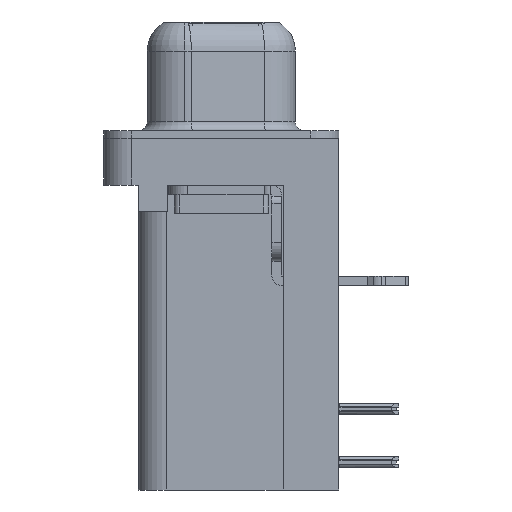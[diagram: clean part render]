
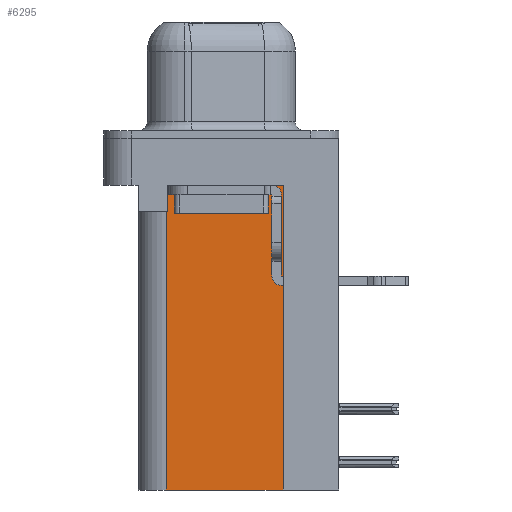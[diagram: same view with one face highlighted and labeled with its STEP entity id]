
A CAD part, left-side view. The second image highlights one B-rep face of the part: STEP entity #6295.
In plain terms, the highlighted planar face has unit normal (-1, 0, 0).
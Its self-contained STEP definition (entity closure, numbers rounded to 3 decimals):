
#154 = CARTESIAN_POINT ( 'NONE',  ( 3.7, -3.295, -2.5 ) ) ;
#504 = EDGE_LOOP ( 'NONE', ( #3798, #9496, #5287, #16333, #21993, #24759 ) ) ;
#3168 = LINE ( 'NONE', #14290, #3319 ) ;
#3319 = VECTOR ( 'NONE', #4103, 1000. ) ;
#3667 = DIRECTION ( 'NONE',  ( 0., 0., 1. ) ) ;
#3798 = ORIENTED_EDGE ( 'NONE', *, *, #9376, .T. ) ;
#4103 = DIRECTION ( 'NONE',  ( 0., 0., -1. ) ) ;
#4229 = VECTOR ( 'NONE', #3667, 1000. ) ;
#4260 = LINE ( 'NONE', #21083, #4229 ) ;
#4864 = LINE ( 'NONE', #24770, #4966 ) ;
#4966 = VECTOR ( 'NONE', #10086, 1000. ) ;
#5287 = ORIENTED_EDGE ( 'NONE', *, *, #19517, .T. ) ;
#5341 = VERTEX_POINT ( 'NONE', #17234 ) ;
#5357 = DIRECTION ( 'NONE',  ( 0., 1., 0. ) ) ;
#5976 = VERTEX_POINT ( 'NONE', #17710 ) ;
#6295 = ADVANCED_FACE ( 'NONE', ( #31057 ), #18889, .F. ) ;
#7734 = LINE ( 'NONE', #14561, #7979 ) ;
#7979 = VECTOR ( 'NONE', #31068, 1000. ) ;
#8431 = CARTESIAN_POINT ( 'NONE',  ( 3.7, 2.925, -3.9 ) ) ;
#9376 = EDGE_CURVE ( 'NONE', #12855, #23977, #10350, .T. ) ;
#9426 = DIRECTION ( 'NONE',  ( 0., 1., 0. ) ) ;
#9496 = ORIENTED_EDGE ( 'NONE', *, *, #18455, .T. ) ;
#10086 = DIRECTION ( 'NONE',  ( 0., 1., 0. ) ) ;
#10314 = VECTOR ( 'NONE', #5357, 1000. ) ;
#10350 = LINE ( 'NONE', #154, #10314 ) ;
#10352 = VERTEX_POINT ( 'NONE', #30588 ) ;
#10585 = AXIS2_PLACEMENT_3D ( 'NONE', #18451, #18413, #18351 ) ;
#12092 = CARTESIAN_POINT ( 'NONE',  ( 3.7, -3.295, -2.5 ) ) ;
#12855 = VERTEX_POINT ( 'NONE', #12092 ) ;
#14290 = CARTESIAN_POINT ( 'NONE',  ( 3.7, 2.895, -3.9 ) ) ;
#14390 = EDGE_CURVE ( 'NONE', #5341, #29382, #4260, .T. ) ;
#14561 = CARTESIAN_POINT ( 'NONE',  ( 3.7, -3.295, -18.76 ) ) ;
#16333 = ORIENTED_EDGE ( 'NONE', *, *, #14390, .F. ) ;
#16865 = CARTESIAN_POINT ( 'NONE',  ( 3.7, 0., -3.9 ) ) ;
#17234 = CARTESIAN_POINT ( 'NONE',  ( 3.7, 2.925, -18.76 ) ) ;
#17710 = CARTESIAN_POINT ( 'NONE',  ( 3.7, 2.895, -3.9 ) ) ;
#17921 = EDGE_CURVE ( 'NONE', #10352, #12855, #7734, .T. ) ;
#18206 = CARTESIAN_POINT ( 'NONE',  ( 3.7, 2.895, -2.5 ) ) ;
#18351 = DIRECTION ( 'NONE',  ( 0., 1., 0. ) ) ;
#18413 = DIRECTION ( 'NONE',  ( 1., 0., 0. ) ) ;
#18451 = CARTESIAN_POINT ( 'NONE',  ( 3.7, -3.295, -18.76 ) ) ;
#18455 = EDGE_CURVE ( 'NONE', #23977, #5976, #3168, .T. ) ;
#18889 = PLANE ( 'NONE',  #10585 ) ;
#19517 = EDGE_CURVE ( 'NONE', #5976, #29382, #29554, .T. ) ;
#20432 = VECTOR ( 'NONE', #9426, 1000. ) ;
#21083 = CARTESIAN_POINT ( 'NONE',  ( 3.7, 2.925, -18.76 ) ) ;
#21993 = ORIENTED_EDGE ( 'NONE', *, *, #30563, .F. ) ;
#23977 = VERTEX_POINT ( 'NONE', #18206 ) ;
#24759 = ORIENTED_EDGE ( 'NONE', *, *, #17921, .T. ) ;
#24770 = CARTESIAN_POINT ( 'NONE',  ( 3.7, -3.295, -18.76 ) ) ;
#29382 = VERTEX_POINT ( 'NONE', #8431 ) ;
#29554 = LINE ( 'NONE', #16865, #20432 ) ;
#30563 = EDGE_CURVE ( 'NONE', #10352, #5341, #4864, .T. ) ;
#30588 = CARTESIAN_POINT ( 'NONE',  ( 3.7, -3.295, -18.76 ) ) ;
#31057 = FACE_OUTER_BOUND ( 'NONE', #504, .T. ) ;
#31068 = DIRECTION ( 'NONE',  ( 0., 0., 1. ) ) ;
